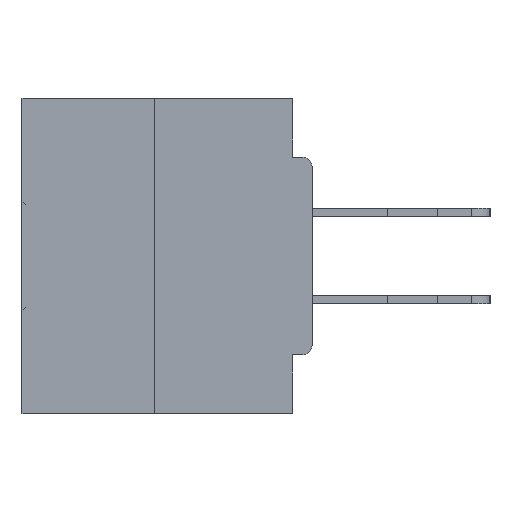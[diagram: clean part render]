
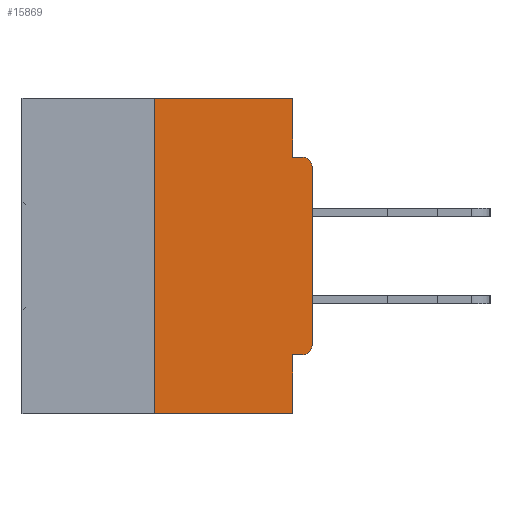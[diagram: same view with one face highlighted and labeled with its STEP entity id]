
A CAD part, left-side view. The second image highlights one B-rep face of the part: STEP entity #15869.
In plain terms, the highlighted planar face has unit normal (-1, 0, 0).
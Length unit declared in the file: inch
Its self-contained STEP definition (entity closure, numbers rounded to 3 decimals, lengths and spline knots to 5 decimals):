
#136 = EDGE_CURVE ( 'NONE', #20221, #17525, #8343, .T. ) ;
#417 = CARTESIAN_POINT ( 'NONE',  ( 0., 0., -0.4065 ) ) ;
#704 = DIRECTION ( 'NONE',  ( -1., 0., 0. ) ) ;
#768 = EDGE_CURVE ( 'NONE', #1330, #20221, #22375, .T. ) ;
#1330 = VERTEX_POINT ( 'NONE', #34172 ) ;
#1525 = DIRECTION ( 'NONE',  ( 0., -1., 0. ) ) ;
#1803 = DIRECTION ( 'NONE',  ( 0., 0., -1. ) ) ;
#2056 = VERTEX_POINT ( 'NONE', #7088 ) ;
#2565 = CARTESIAN_POINT ( 'NONE',  ( 0., 0.031, -0.0935 ) ) ;
#3696 = CARTESIAN_POINT ( 'NONE',  ( 0., 0.25, 0. ) ) ;
#4253 = ORIENTED_EDGE ( 'NONE', *, *, #31254, .T. ) ;
#5633 = CARTESIAN_POINT ( 'NONE',  ( 0., 0., -0.1085 ) ) ;
#5716 = CIRCLE ( 'NONE', #43476, 0.015 ) ;
#6645 = VERTEX_POINT ( 'NONE', #5633 ) ;
#7088 = CARTESIAN_POINT ( 'NONE',  ( 0., 0.031, -0.5 ) ) ;
#7090 = VERTEX_POINT ( 'NONE', #26719 ) ;
#8210 = VECTOR ( 'NONE', #36273, 39.37008 ) ;
#8343 = LINE ( 'NONE', #14943, #9624 ) ;
#8933 = CARTESIAN_POINT ( 'NONE',  ( 0., 0., -0.3915 ) ) ;
#8967 = CARTESIAN_POINT ( 'NONE',  ( 0., 0.031, 0. ) ) ;
#9354 = CARTESIAN_POINT ( 'NONE',  ( 0., 0.015, -0.0935 ) ) ;
#9624 = VECTOR ( 'NONE', #1525, 39.37008 ) ;
#9671 = LINE ( 'NONE', #24208, #41493 ) ;
#9921 = DIRECTION ( 'NONE',  ( 0., 0., 1. ) ) ;
#10147 = LINE ( 'NONE', #17405, #14533 ) ;
#10512 = DIRECTION ( 'NONE',  ( 0., 0., 1. ) ) ;
#11489 = ORIENTED_EDGE ( 'NONE', *, *, #768, .F. ) ;
#11521 = ORIENTED_EDGE ( 'NONE', *, *, #32306, .F. ) ;
#12094 = EDGE_CURVE ( 'NONE', #15560, #1330, #9671, .T. ) ;
#13798 = DIRECTION ( 'NONE',  ( 0., 0., -1. ) ) ;
#14533 = VECTOR ( 'NONE', #30855, 39.37008 ) ;
#14943 = CARTESIAN_POINT ( 'NONE',  ( 0., 0., -0.0935 ) ) ;
#15560 = VERTEX_POINT ( 'NONE', #31818 ) ;
#15869 = ADVANCED_FACE ( 'NONE', ( #20140 ), #20373, .F. ) ;
#16079 = VECTOR ( 'NONE', #26460, 39.37008 ) ;
#16123 = DIRECTION ( 'NONE',  ( -1., 0., 0. ) ) ;
#17184 = ORIENTED_EDGE ( 'NONE', *, *, #22155, .T. ) ;
#17300 = LINE ( 'NONE', #417, #35190 ) ;
#17405 = CARTESIAN_POINT ( 'NONE',  ( 0., 0.031, -0.5 ) ) ;
#17525 = VERTEX_POINT ( 'NONE', #9354 ) ;
#17915 = DIRECTION ( 'NONE',  ( 0., 1., 0. ) ) ;
#18631 = CARTESIAN_POINT ( 'NONE',  ( 0., 0.015, -0.3915 ) ) ;
#19308 = AXIS2_PLACEMENT_3D ( 'NONE', #18631, #704, #32321 ) ;
#19909 = CARTESIAN_POINT ( 'NONE',  ( 0., 0., 0. ) ) ;
#20140 = FACE_OUTER_BOUND ( 'NONE', #38886, .T. ) ;
#20221 = VERTEX_POINT ( 'NONE', #2565 ) ;
#20222 = VERTEX_POINT ( 'NONE', #8933 ) ;
#20373 = PLANE ( 'NONE',  #24168 ) ;
#22155 = EDGE_CURVE ( 'NONE', #6645, #17525, #5716, .T. ) ;
#22375 = LINE ( 'NONE', #8967, #8210 ) ;
#23404 = EDGE_CURVE ( 'NONE', #26230, #2056, #10147, .T. ) ;
#23838 = ORIENTED_EDGE ( 'NONE', *, *, #12094, .F. ) ;
#24168 = AXIS2_PLACEMENT_3D ( 'NONE', #44953, #31095, #13798 ) ;
#24208 = CARTESIAN_POINT ( 'NONE',  ( 0., 0.46, 0. ) ) ;
#26230 = VERTEX_POINT ( 'NONE', #35297 ) ;
#26448 = LINE ( 'NONE', #3696, #28175 ) ;
#26460 = DIRECTION ( 'NONE',  ( 0., -1., 0. ) ) ;
#26719 = CARTESIAN_POINT ( 'NONE',  ( 0., 0.015, -0.4065 ) ) ;
#28175 = VECTOR ( 'NONE', #10512, 39.37008 ) ;
#28670 = ORIENTED_EDGE ( 'NONE', *, *, #29737, .T. ) ;
#28996 = EDGE_CURVE ( 'NONE', #29873, #2056, #36493, .T. ) ;
#29737 = EDGE_CURVE ( 'NONE', #20222, #6645, #37224, .T. ) ;
#29873 = VERTEX_POINT ( 'NONE', #29960 ) ;
#29960 = CARTESIAN_POINT ( 'NONE',  ( 0., 0.25, -0.5 ) ) ;
#30117 = CARTESIAN_POINT ( 'NONE',  ( 0., 0.46, -0.5 ) ) ;
#30855 = DIRECTION ( 'NONE',  ( 0., 0., -1. ) ) ;
#31095 = DIRECTION ( 'NONE',  ( 1., 0., 0. ) ) ;
#31254 = EDGE_CURVE ( 'NONE', #7090, #20222, #38939, .T. ) ;
#31818 = CARTESIAN_POINT ( 'NONE',  ( 0., 0.25, 0. ) ) ;
#32306 = EDGE_CURVE ( 'NONE', #29873, #15560, #26448, .T. ) ;
#32321 = DIRECTION ( 'NONE',  ( 0., 0., -1. ) ) ;
#34172 = CARTESIAN_POINT ( 'NONE',  ( 0., 0.031, 0. ) ) ;
#34770 = ORIENTED_EDGE ( 'NONE', *, *, #23404, .F. ) ;
#35190 = VECTOR ( 'NONE', #17915, 39.37008 ) ;
#35297 = CARTESIAN_POINT ( 'NONE',  ( 0., 0.031, -0.4065 ) ) ;
#35870 = ORIENTED_EDGE ( 'NONE', *, *, #136, .F. ) ;
#36273 = DIRECTION ( 'NONE',  ( 0., 0., -1. ) ) ;
#36493 = LINE ( 'NONE', #30117, #16079 ) ;
#37224 = LINE ( 'NONE', #19909, #43741 ) ;
#38082 = DIRECTION ( 'NONE',  ( 0., -1., 0. ) ) ;
#38886 = EDGE_LOOP ( 'NONE', ( #23838, #11521, #42936, #34770, #43130, #4253, #28670, #17184, #35870, #11489 ) ) ;
#38939 = CIRCLE ( 'NONE', #19308, 0.015 ) ;
#40021 = CARTESIAN_POINT ( 'NONE',  ( 0., 0.015, -0.1085 ) ) ;
#41196 = EDGE_CURVE ( 'NONE', #7090, #26230, #17300, .T. ) ;
#41493 = VECTOR ( 'NONE', #38082, 39.37008 ) ;
#42936 = ORIENTED_EDGE ( 'NONE', *, *, #28996, .T. ) ;
#43130 = ORIENTED_EDGE ( 'NONE', *, *, #41196, .F. ) ;
#43476 = AXIS2_PLACEMENT_3D ( 'NONE', #40021, #16123, #1803 ) ;
#43741 = VECTOR ( 'NONE', #9921, 39.37008 ) ;
#44953 = CARTESIAN_POINT ( 'NONE',  ( 0., 0.46, 0. ) ) ;
